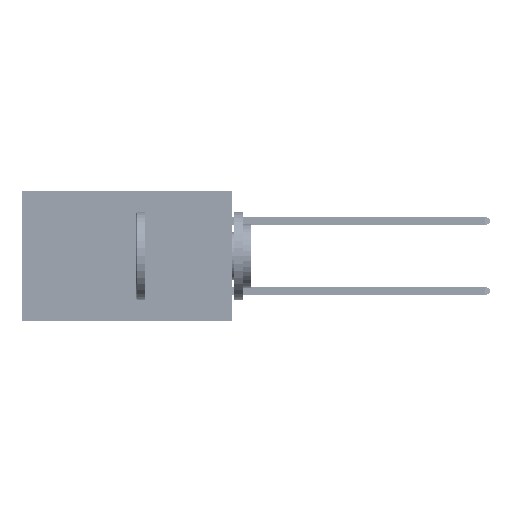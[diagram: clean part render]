
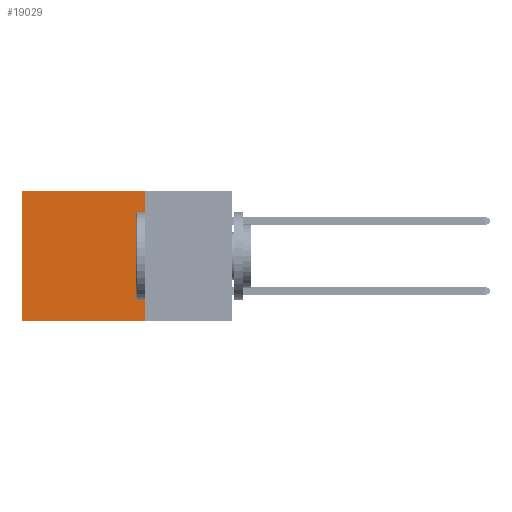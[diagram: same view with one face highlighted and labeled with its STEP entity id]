
A CAD part, left-side view. The second image highlights one B-rep face of the part: STEP entity #19029.
In plain terms, the highlighted planar face has unit normal (-1, 0, 0).
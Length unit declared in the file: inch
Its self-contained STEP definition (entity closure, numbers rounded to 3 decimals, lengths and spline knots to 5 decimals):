
#218 = EDGE_CURVE ( 'NONE', #48541, #49561, #39718, .T. ) ;
#1448 = CARTESIAN_POINT ( 'NONE',  ( 0.2875, 0.25, -0.37 ) ) ;
#1912 = EDGE_CURVE ( 'NONE', #11551, #43788, #14422, .T. ) ;
#1937 = DIRECTION ( 'NONE',  ( 0., 1., 0. ) ) ;
#7701 = VECTOR ( 'NONE', #42149, 39.37008 ) ;
#9901 = CARTESIAN_POINT ( 'NONE',  ( 0.2875, 0.6, -0.37 ) ) ;
#11404 = ORIENTED_EDGE ( 'NONE', *, *, #49606, .T. ) ;
#11461 = ORIENTED_EDGE ( 'NONE', *, *, #218, .T. ) ;
#11551 = VERTEX_POINT ( 'NONE', #41476 ) ;
#11598 = LINE ( 'NONE', #1448, #39389 ) ;
#12628 = CARTESIAN_POINT ( 'NONE',  ( 0.2875, 0.25, -0.37 ) ) ;
#13495 = CARTESIAN_POINT ( 'NONE',  ( 0.2875, 0.6, 0. ) ) ;
#14422 = LINE ( 'NONE', #22446, #16890 ) ;
#16890 = VECTOR ( 'NONE', #35454, 39.37008 ) ;
#18122 = LINE ( 'NONE', #42837, #7701 ) ;
#19029 = ADVANCED_FACE ( 'NONE', ( #43750 ), #26638, .F. ) ;
#20780 = AXIS2_PLACEMENT_3D ( 'NONE', #38230, #22474, #38568 ) ;
#21176 = EDGE_LOOP ( 'NONE', ( #11461, #44526, #40808, #11404 ) ) ;
#22446 = CARTESIAN_POINT ( 'NONE',  ( 0.2875, 0.25, 0. ) ) ;
#22474 = DIRECTION ( 'NONE',  ( 1., 0., 0. ) ) ;
#26638 = PLANE ( 'NONE',  #20780 ) ;
#26768 = CARTESIAN_POINT ( 'NONE',  ( 0.2875, 0.6, 0. ) ) ;
#27342 = EDGE_CURVE ( 'NONE', #43788, #49561, #11598, .T. ) ;
#35454 = DIRECTION ( 'NONE',  ( 0., 0., -1. ) ) ;
#38230 = CARTESIAN_POINT ( 'NONE',  ( 0.2875, 0.25, 0. ) ) ;
#38568 = DIRECTION ( 'NONE',  ( 0., 0., -1. ) ) ;
#39389 = VECTOR ( 'NONE', #1937, 39.37008 ) ;
#39718 = LINE ( 'NONE', #13495, #40309 ) ;
#40309 = VECTOR ( 'NONE', #49027, 39.37008 ) ;
#40808 = ORIENTED_EDGE ( 'NONE', *, *, #1912, .F. ) ;
#41476 = CARTESIAN_POINT ( 'NONE',  ( 0.2875, 0.25, 0. ) ) ;
#42149 = DIRECTION ( 'NONE',  ( 0., 1., 0. ) ) ;
#42837 = CARTESIAN_POINT ( 'NONE',  ( 0.2875, 0.25, 0. ) ) ;
#43750 = FACE_OUTER_BOUND ( 'NONE', #21176, .T. ) ;
#43788 = VERTEX_POINT ( 'NONE', #12628 ) ;
#44526 = ORIENTED_EDGE ( 'NONE', *, *, #27342, .F. ) ;
#48541 = VERTEX_POINT ( 'NONE', #26768 ) ;
#49027 = DIRECTION ( 'NONE',  ( 0., 0., -1. ) ) ;
#49561 = VERTEX_POINT ( 'NONE', #9901 ) ;
#49606 = EDGE_CURVE ( 'NONE', #11551, #48541, #18122, .T. ) ;
